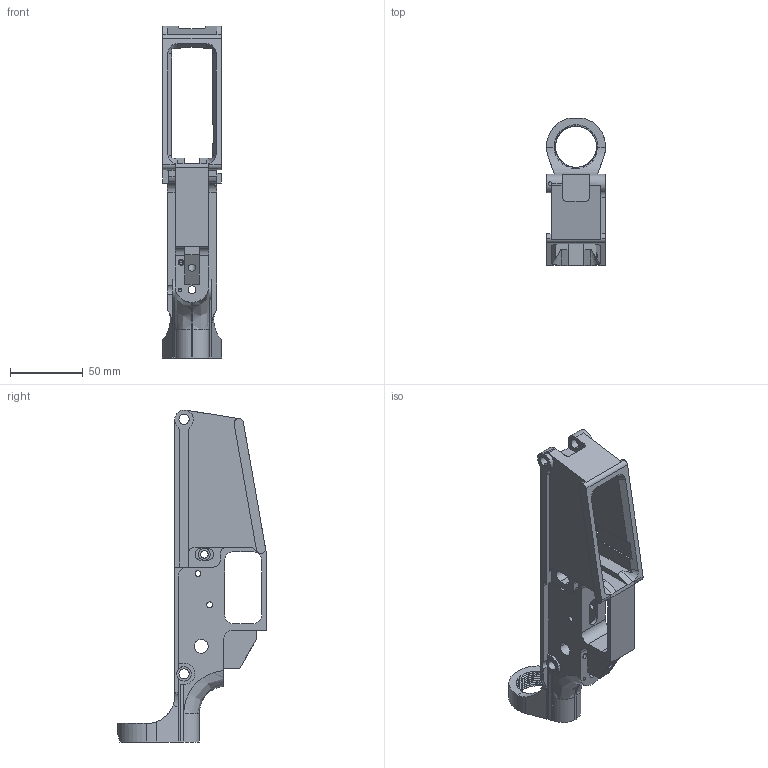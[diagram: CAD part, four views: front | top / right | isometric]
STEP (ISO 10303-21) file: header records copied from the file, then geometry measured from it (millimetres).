
FILE_DESCRIPTION (( 'STEP AP214' ), '1' );
FILE_NAME ('LR308 v1.2.STEP', '2016-04-26T18:03:48', ( '' ), ( '' ), 'SwSTEP 2.0', 'SolidWorks 2013', '' );
FILE_SCHEMA (( 'AUTOMOTIVE_DESIGN' ));
Length unit declared in the file: inch
Products named in the file (1): LR308 v1.2
Bounding box: 40.51 x 101.6 x 227.84 mm (x, y, z)
Volume: 129762.5 mm3; surface area: 64236.7 mm2
Topology: 1 solids, 1 shells, 305 faces, 904 edges, 595 vertices
Faces by surface type: cylinder 139, plane 131, bspline 22, cone 13
Entity records: 21096 total; most frequent: CARTESIAN_POINT 13088, ORIENTED_EDGE 1800, DIRECTION 1538, EDGE_CURVE 900, VERTEX_POINT 595, AXIS2_PLACEMENT_3D 523, VECTOR 492, LINE 492
